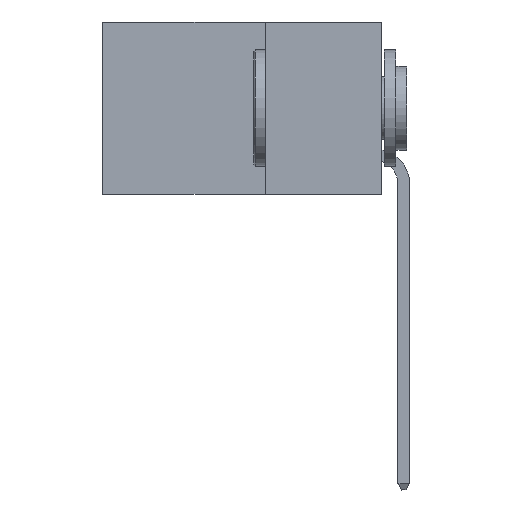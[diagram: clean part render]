
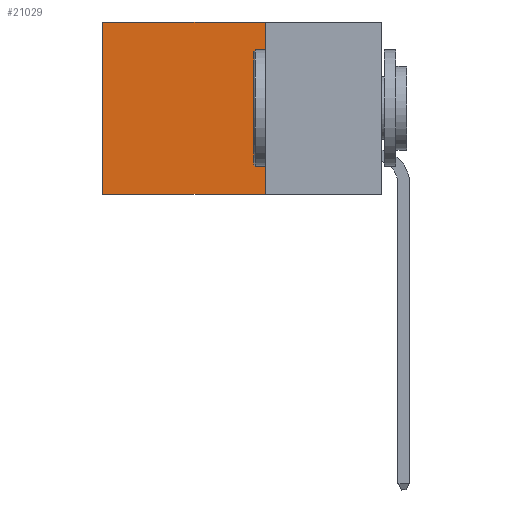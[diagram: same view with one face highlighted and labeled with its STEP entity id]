
A CAD part, left-side view. The second image highlights one B-rep face of the part: STEP entity #21029.
In plain terms, the highlighted planar face has unit normal (-1, 0, 0).
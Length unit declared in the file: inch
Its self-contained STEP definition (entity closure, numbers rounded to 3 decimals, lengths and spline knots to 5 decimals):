
#114 = CARTESIAN_POINT ( 'NONE',  ( 0.2875, 0.25, 0. ) ) ;
#290 = ORIENTED_EDGE ( 'NONE', *, *, #11510, .F. ) ;
#2098 = FACE_OUTER_BOUND ( 'NONE', #17704, .T. ) ;
#2996 = VECTOR ( 'NONE', #19516, 39.37008 ) ;
#4822 = EDGE_CURVE ( 'NONE', #16357, #26799, #6063, .T. ) ;
#5307 = EDGE_CURVE ( 'NONE', #6029, #16357, #12974, .T. ) ;
#5628 = CARTESIAN_POINT ( 'NONE',  ( 0.2875, 0.25, -0.37 ) ) ;
#6029 = VERTEX_POINT ( 'NONE', #114 ) ;
#6063 = LINE ( 'NONE', #11634, #19675 ) ;
#7313 = DIRECTION ( 'NONE',  ( 0., 0., -1. ) ) ;
#7741 = CARTESIAN_POINT ( 'NONE',  ( 0.2875, 0.25, 0. ) ) ;
#8380 = CARTESIAN_POINT ( 'NONE',  ( 0.2875, 0.25, -0.37 ) ) ;
#8484 = AXIS2_PLACEMENT_3D ( 'NONE', #7741, #18009, #15978 ) ;
#8649 = VECTOR ( 'NONE', #17330, 39.37008 ) ;
#9777 = PLANE ( 'NONE',  #8484 ) ;
#10742 = ORIENTED_EDGE ( 'NONE', *, *, #4822, .T. ) ;
#11510 = EDGE_CURVE ( 'NONE', #6029, #21682, #16902, .T. ) ;
#11634 = CARTESIAN_POINT ( 'NONE',  ( 0.2875, 0.6, 0. ) ) ;
#11785 = CARTESIAN_POINT ( 'NONE',  ( 0.2875, 0.6, -0.37 ) ) ;
#12974 = LINE ( 'NONE', #25761, #2996 ) ;
#15883 = VECTOR ( 'NONE', #7313, 39.37008 ) ;
#15978 = DIRECTION ( 'NONE',  ( 0., 0., -1. ) ) ;
#16357 = VERTEX_POINT ( 'NONE', #18671 ) ;
#16902 = LINE ( 'NONE', #17954, #15883 ) ;
#17330 = DIRECTION ( 'NONE',  ( 0., 1., 0. ) ) ;
#17704 = EDGE_LOOP ( 'NONE', ( #10742, #20161, #290, #19958 ) ) ;
#17954 = CARTESIAN_POINT ( 'NONE',  ( 0.2875, 0.25, 0. ) ) ;
#18009 = DIRECTION ( 'NONE',  ( 1., 0., 0. ) ) ;
#18671 = CARTESIAN_POINT ( 'NONE',  ( 0.2875, 0.6, 0. ) ) ;
#19516 = DIRECTION ( 'NONE',  ( 0., 1., 0. ) ) ;
#19675 = VECTOR ( 'NONE', #19938, 39.37008 ) ;
#19938 = DIRECTION ( 'NONE',  ( 0., 0., -1. ) ) ;
#19958 = ORIENTED_EDGE ( 'NONE', *, *, #5307, .T. ) ;
#20161 = ORIENTED_EDGE ( 'NONE', *, *, #24182, .F. ) ;
#21029 = ADVANCED_FACE ( 'NONE', ( #2098 ), #9777, .F. ) ;
#21682 = VERTEX_POINT ( 'NONE', #5628 ) ;
#23296 = LINE ( 'NONE', #8380, #8649 ) ;
#24182 = EDGE_CURVE ( 'NONE', #21682, #26799, #23296, .T. ) ;
#25761 = CARTESIAN_POINT ( 'NONE',  ( 0.2875, 0.25, 0. ) ) ;
#26799 = VERTEX_POINT ( 'NONE', #11785 ) ;
